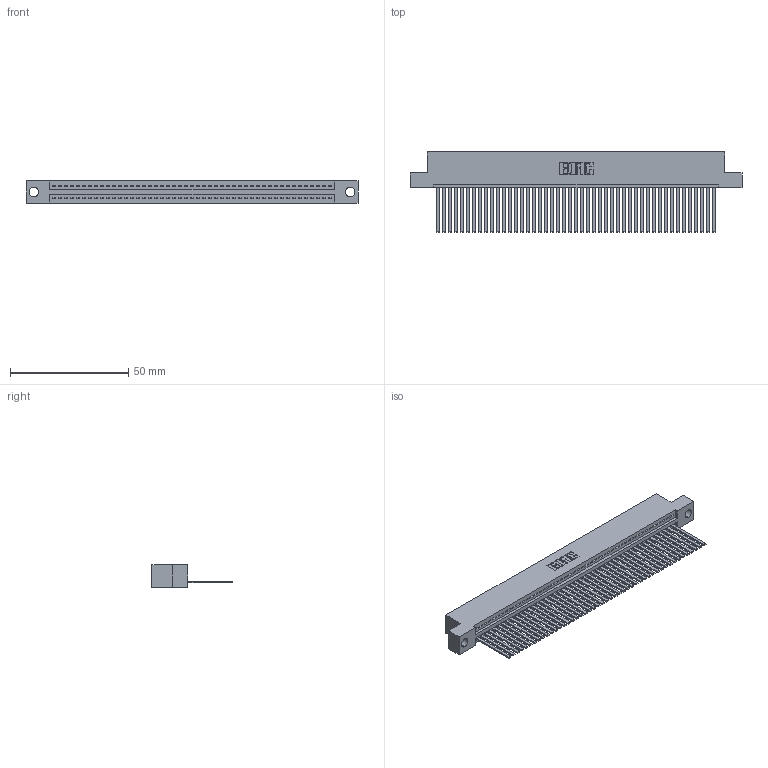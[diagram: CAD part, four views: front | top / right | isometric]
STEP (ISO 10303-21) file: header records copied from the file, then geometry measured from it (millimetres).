
FILE_DESCRIPTION (( 'STEP AP203' ), '1' );
FILE_NAME ('395-047-544-104.STEP', '2021-05-31T15:15:46', ( '' ), ( '' ), 'SwSTEP 2.0', 'SolidWorks 2020', '' );
FILE_SCHEMA (( 'CONFIG_CONTROL_DESIGN' ));
Length unit declared in the file: inch
Products named in the file (3): 345-292-001_345-293-144; 395-047-544-104; 345 Part_Flush Mounting Lugs - 0.156 Dia-TI
Assembly tree (48 placements, depth 2):
  395-047-544-104
    345 Part_Flush Mounting Lugs - 0.156 Dia-TI
    345-292-001_345-293-144  x47
Bounding box: 140.59 x 33.96 x 9.4 mm (x, y, z)
Volume: 13832.6 mm3; surface area: 19926.8 mm2
Topology: 48 solids, 48 shells, 2584 faces, 7803 edges, 5138 vertices
Faces by surface type: plane 1786, cylinder 798
Entity records: 34935 total; most frequent: CARTESIAN_POINT 6059, ORIENTED_EDGE 6038, DIRECTION 5281, EDGE_CURVE 3019, LINE 2703, VECTOR 2703, VERTEX_POINT 2010, AXIS2_PLACEMENT_3D 1289
